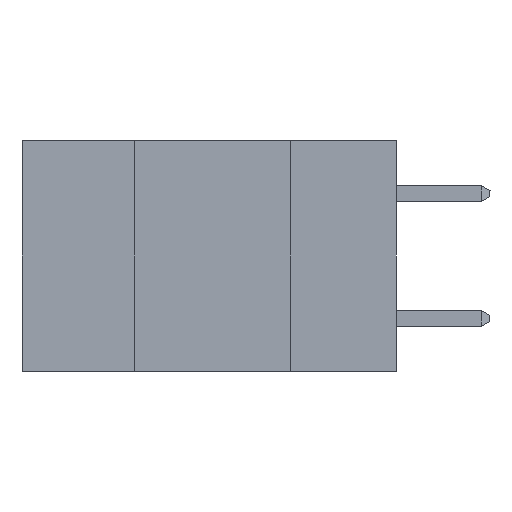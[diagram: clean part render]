
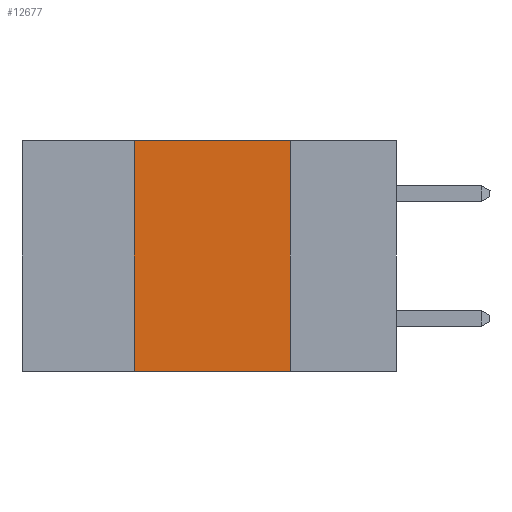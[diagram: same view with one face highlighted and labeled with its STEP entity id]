
A CAD part, left-side view. The second image highlights one B-rep face of the part: STEP entity #12677.
In plain terms, the highlighted planar face has unit normal (-1, 0, 0).
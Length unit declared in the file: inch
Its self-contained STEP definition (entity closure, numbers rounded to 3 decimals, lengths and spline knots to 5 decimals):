
#2940 = LINE ( 'NONE', #27219, #7793 ) ;
#3285 = LINE ( 'NONE', #8341, #8888 ) ;
#4524 = CARTESIAN_POINT ( 'NONE',  ( 0., 0.42, 0. ) ) ;
#5597 = VERTEX_POINT ( 'NONE', #7751 ) ;
#6321 = ORIENTED_EDGE ( 'NONE', *, *, #15813, .T. ) ;
#6338 = VERTEX_POINT ( 'NONE', #6586 ) ;
#6586 = CARTESIAN_POINT ( 'NONE',  ( 0., 0.17, 0. ) ) ;
#7423 = EDGE_CURVE ( 'NONE', #5597, #6338, #2940, .T. ) ;
#7751 = CARTESIAN_POINT ( 'NONE',  ( 0., 0.42, 0. ) ) ;
#7793 = VECTOR ( 'NONE', #26778, 39.37008 ) ;
#8341 = CARTESIAN_POINT ( 'NONE',  ( 0., 0.17, 0. ) ) ;
#8599 = CARTESIAN_POINT ( 'NONE',  ( 0., 0.17, -0.37 ) ) ;
#8888 = VECTOR ( 'NONE', #22894, 39.37008 ) ;
#11329 = LINE ( 'NONE', #21871, #16255 ) ;
#11625 = ORIENTED_EDGE ( 'NONE', *, *, #7423, .F. ) ;
#11980 = PLANE ( 'NONE',  #20092 ) ;
#12598 = EDGE_CURVE ( 'NONE', #16032, #5597, #19993, .T. ) ;
#12677 = ADVANCED_FACE ( 'NONE', ( #19229 ), #11980, .F. ) ;
#13561 = VECTOR ( 'NONE', #26356, 39.37008 ) ;
#14292 = VERTEX_POINT ( 'NONE', #8599 ) ;
#15813 = EDGE_CURVE ( 'NONE', #16032, #14292, #11329, .T. ) ;
#16032 = VERTEX_POINT ( 'NONE', #22617 ) ;
#16255 = VECTOR ( 'NONE', #24352, 39.37008 ) ;
#16850 = DIRECTION ( 'NONE',  ( 0., 0., -1. ) ) ;
#18068 = EDGE_CURVE ( 'NONE', #6338, #14292, #3285, .T. ) ;
#18488 = ORIENTED_EDGE ( 'NONE', *, *, #12598, .F. ) ;
#19204 = CARTESIAN_POINT ( 'NONE',  ( 0., 0.6, 0. ) ) ;
#19229 = FACE_OUTER_BOUND ( 'NONE', #29675, .T. ) ;
#19993 = LINE ( 'NONE', #4524, #13561 ) ;
#20092 = AXIS2_PLACEMENT_3D ( 'NONE', #19204, #31432, #16850 ) ;
#21107 = ORIENTED_EDGE ( 'NONE', *, *, #18068, .F. ) ;
#21871 = CARTESIAN_POINT ( 'NONE',  ( 0., 0.6, -0.37 ) ) ;
#22617 = CARTESIAN_POINT ( 'NONE',  ( 0., 0.42, -0.37 ) ) ;
#22894 = DIRECTION ( 'NONE',  ( 0., 0., -1. ) ) ;
#24352 = DIRECTION ( 'NONE',  ( 0., -1., 0. ) ) ;
#26356 = DIRECTION ( 'NONE',  ( 0., 0., 1. ) ) ;
#26778 = DIRECTION ( 'NONE',  ( 0., -1., 0. ) ) ;
#27219 = CARTESIAN_POINT ( 'NONE',  ( 0., 0.6, 0. ) ) ;
#29675 = EDGE_LOOP ( 'NONE', ( #21107, #11625, #18488, #6321 ) ) ;
#31432 = DIRECTION ( 'NONE',  ( 1., 0., 0. ) ) ;
